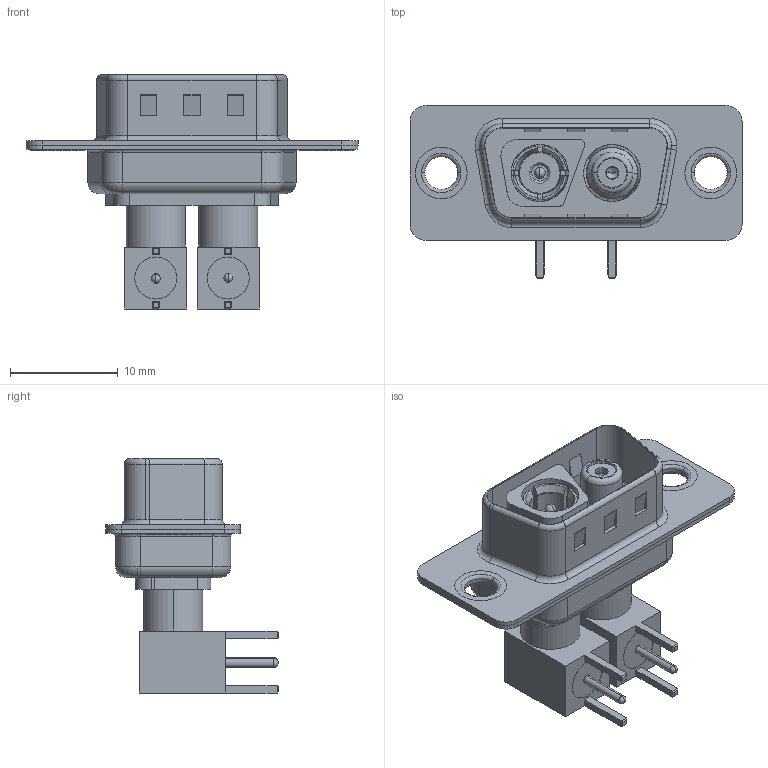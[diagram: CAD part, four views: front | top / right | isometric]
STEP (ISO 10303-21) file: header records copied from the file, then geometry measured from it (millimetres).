
FILE_DESCRIPTION (( 'STEP AP203' ), '1' );
FILE_NAME ('629-2WK2240-5N1.STEP', '2022-05-04T23:13:26', ( '' ), ( '' ), 'SwSTEP 2.0', 'SolidWorks 2020', '' );
FILE_SCHEMA (( 'CONFIG_CONTROL_DESIGN' ));
Length unit declared in the file: millimetre
Products named in the file (17): 629Combo Thru Hole Rivet; Insulator Socket 2; Locking Collar; 629Combo Housing_2WK2; Pin_RA; Socket_RA; Insulator Pin_Straight PC Tail; Co-Ax Plug Assy_RA; Insulator RA Pin; Co-Ax Plug_RA PC Tail; 629-2WK2240-5N1; Co-Ax Jack Assy_RA; RA Back Shell; 629Combo Shell Rear_09 Contacts; Insulator Socket; Co-Ax Jack_RA PC Tail; 629Combo Shell Front_09 Contacts
Assembly tree (20 placements, depth 3):
  629-2WK2240-5N1
    629Combo Housing_2WK2
    629Combo Shell Rear_09 Contacts
    629Combo Shell Front_09 Contacts
    629Combo Thru Hole Rivet  x2
    Co-Ax Plug Assy_RA
      Co-Ax Plug_RA PC Tail
      Insulator Pin_Straight PC Tail
      Pin_RA
      Locking Collar
      RA Back Shell
      Insulator RA Pin
    Co-Ax Jack Assy_RA
      Co-Ax Jack_RA PC Tail
      Insulator Socket
      Insulator Socket 2
      Locking Collar
      Socket_RA
      RA Back Shell
      Insulator RA Pin
Bounding box: 30.8 x 16 x 21.71 mm (x, y, z)
Volume: 1916 mm3; surface area: 5454.3 mm2
Topology: 18 solids, 18 shells, 608 faces, 1448 edges, 900 vertices
Faces by surface type: cylinder 250, plane 236, torus 70, cone 44, sphere 6, bspline 2
Entity records: 17641 total; most frequent: CARTESIAN_POINT 2949, DIRECTION 2904, ORIENTED_EDGE 2510, EDGE_CURVE 1255, AXIS2_PLACEMENT_3D 1143, VERTEX_POINT 791, LINE 618, VECTOR 618
